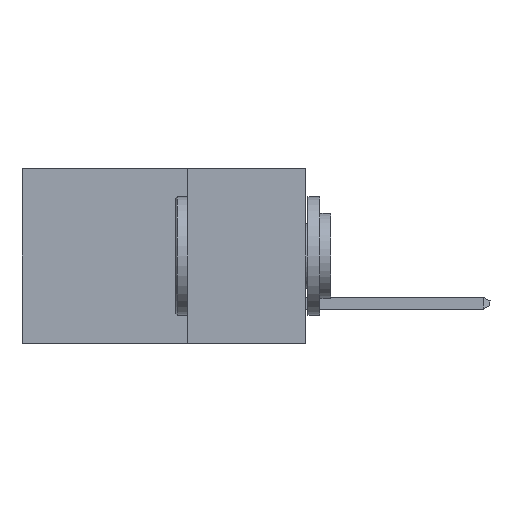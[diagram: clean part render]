
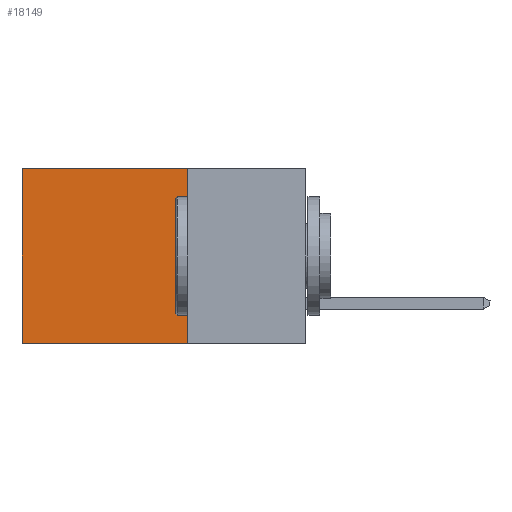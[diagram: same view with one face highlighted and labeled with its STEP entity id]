
A CAD part, left-side view. The second image highlights one B-rep face of the part: STEP entity #18149.
In plain terms, the highlighted planar face has unit normal (-1, 0, 0).
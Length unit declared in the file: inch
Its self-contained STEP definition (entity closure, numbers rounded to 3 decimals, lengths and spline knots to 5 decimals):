
#393 = VECTOR ( 'NONE', #3133, 39.37008 ) ;
#2048 = EDGE_CURVE ( 'NONE', #13960, #23843, #18535, .T. ) ;
#3133 = DIRECTION ( 'NONE',  ( 0., 0., -1. ) ) ;
#3873 = PLANE ( 'NONE',  #15938 ) ;
#5045 = CARTESIAN_POINT ( 'NONE',  ( 0.298, 0.25, -0.37 ) ) ;
#5421 = VECTOR ( 'NONE', #8796, 39.37008 ) ;
#5530 = EDGE_CURVE ( 'NONE', #9286, #23843, #9185, .T. ) ;
#6205 = ORIENTED_EDGE ( 'NONE', *, *, #12521, .T. ) ;
#6947 = VERTEX_POINT ( 'NONE', #11555 ) ;
#7008 = DIRECTION ( 'NONE',  ( 0., 1., 0. ) ) ;
#8169 = VECTOR ( 'NONE', #19777, 39.37008 ) ;
#8796 = DIRECTION ( 'NONE',  ( 0., 1., 0. ) ) ;
#9185 = LINE ( 'NONE', #5045, #5421 ) ;
#9286 = VERTEX_POINT ( 'NONE', #22298 ) ;
#10403 = CARTESIAN_POINT ( 'NONE',  ( 0.298, 0.25, 0. ) ) ;
#10831 = CARTESIAN_POINT ( 'NONE',  ( 0.298, 0.6, 0. ) ) ;
#11401 = CARTESIAN_POINT ( 'NONE',  ( 0.298, 0.25, 0. ) ) ;
#11555 = CARTESIAN_POINT ( 'NONE',  ( 0.298, 0.25, 0. ) ) ;
#12521 = EDGE_CURVE ( 'NONE', #6947, #13960, #17973, .T. ) ;
#13081 = VECTOR ( 'NONE', #7008, 39.37008 ) ;
#13609 = CARTESIAN_POINT ( 'NONE',  ( 0.298, 0.6, 0. ) ) ;
#13960 = VERTEX_POINT ( 'NONE', #13609 ) ;
#14193 = CARTESIAN_POINT ( 'NONE',  ( 0.298, 0.25, 0. ) ) ;
#14593 = ORIENTED_EDGE ( 'NONE', *, *, #2048, .T. ) ;
#15938 = AXIS2_PLACEMENT_3D ( 'NONE', #11401, #17413, #19033 ) ;
#16255 = CARTESIAN_POINT ( 'NONE',  ( 0.298, 0.6, -0.37 ) ) ;
#17031 = EDGE_LOOP ( 'NONE', ( #14593, #22727, #23262, #6205 ) ) ;
#17413 = DIRECTION ( 'NONE',  ( 1., 0., 0. ) ) ;
#17973 = LINE ( 'NONE', #10403, #13081 ) ;
#18149 = ADVANCED_FACE ( 'NONE', ( #18727 ), #3873, .F. ) ;
#18535 = LINE ( 'NONE', #10831, #8169 ) ;
#18727 = FACE_OUTER_BOUND ( 'NONE', #17031, .T. ) ;
#19033 = DIRECTION ( 'NONE',  ( 0., 0., -1. ) ) ;
#19777 = DIRECTION ( 'NONE',  ( 0., 0., -1. ) ) ;
#21373 = EDGE_CURVE ( 'NONE', #6947, #9286, #21765, .T. ) ;
#21765 = LINE ( 'NONE', #14193, #393 ) ;
#22298 = CARTESIAN_POINT ( 'NONE',  ( 0.298, 0.25, -0.37 ) ) ;
#22727 = ORIENTED_EDGE ( 'NONE', *, *, #5530, .F. ) ;
#23262 = ORIENTED_EDGE ( 'NONE', *, *, #21373, .F. ) ;
#23843 = VERTEX_POINT ( 'NONE', #16255 ) ;
